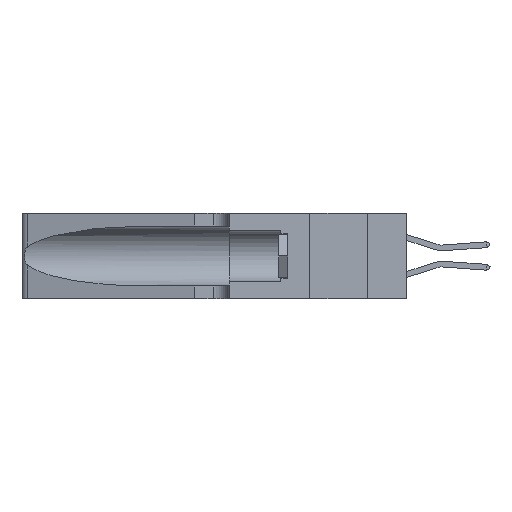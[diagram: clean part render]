
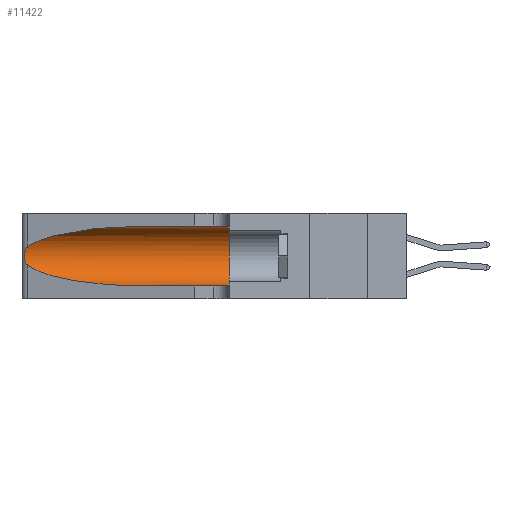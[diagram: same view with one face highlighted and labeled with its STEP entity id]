
A CAD part, left-side view. The second image highlights one B-rep face of the part: STEP entity #11422.
In plain terms, the highlighted cylindrical face has radius 3.308 mm (diameter 6.617 mm), a partial arc.
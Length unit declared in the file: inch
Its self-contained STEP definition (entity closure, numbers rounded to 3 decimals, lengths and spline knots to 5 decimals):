
#431 = CARTESIAN_POINT ( 'NONE',  ( 0.25854, 1.2359, 0.20912 ) ) ;
#1284 = CARTESIAN_POINT ( 'NONE',  ( 0.1305, 0.72297, 0.05475 ) ) ;
#1430 = VERTEX_POINT ( 'NONE', #6978 ) ;
#3313 =( BOUNDED_CURVE ( )  B_SPLINE_CURVE ( 3, ( #6517, #9630, #30344, #12624 ),
 .UNSPECIFIED., .F., .F. ) 
 B_SPLINE_CURVE_WITH_KNOTS ( ( 4, 4 ),
 ( 1.5708, 2.84003 ),
 .UNSPECIFIED. ) 
 CURVE ( )  GEOMETRIC_REPRESENTATION_ITEM ( )  RATIONAL_B_SPLINE_CURVE ( ( 1., 0.87, 0.87, 1. ) ) 
 REPRESENTATION_ITEM ( '' )  );
#3360 = CARTESIAN_POINT ( 'NONE',  ( 0.25487, 1.22718, 0.22369 ) ) ;
#3491 = CARTESIAN_POINT ( 'NONE',  ( 0.26075, 1.23896, 0.19203 ) ) ;
#4408 = B_SPLINE_CURVE_WITH_KNOTS ( 'NONE', 3,
 ( #3360, #15517, #36188, #18493, #431, #21440, #3491, #24396, #6551, #27395, #9664, #30375, #12656, #33358 ),
 .UNSPECIFIED., .F., .F.,
 ( 4, 2, 2, 2, 2, 2, 4 ),
 ( 0., 0.00027, 0.00053, 0.00107, 0.0016, 0.00187, 0.00214 ),
 .UNSPECIFIED. ) ;
#6018 =( BOUNDED_CURVE ( )  B_SPLINE_CURVE ( 3, ( #37023, #16361, #34066, #1284 ),
 .UNSPECIFIED., .F., .T. ) 
 B_SPLINE_CURVE_WITH_KNOTS ( ( 4, 4 ),
 ( 3.44316, 4.71239 ),
 .UNSPECIFIED. ) 
 CURVE ( )  GEOMETRIC_REPRESENTATION_ITEM ( )  RATIONAL_B_SPLINE_CURVE ( ( 1., 0.87, 0.87, 1. ) ) 
 REPRESENTATION_ITEM ( '' )  );
#6517 = CARTESIAN_POINT ( 'NONE',  ( 0.1305, 0.72297, 0.31525 ) ) ;
#6551 = CARTESIAN_POINT ( 'NONE',  ( 0.26017, 1.23833, 0.17102 ) ) ;
#6978 = CARTESIAN_POINT ( 'NONE',  ( 0.1305, 0.35, 0.05475 ) ) ;
#7265 = DIRECTION ( 'NONE',  ( 0., -1., 0. ) ) ;
#9630 = CARTESIAN_POINT ( 'NONE',  ( 0.18966, 0.96281, 0.31525 ) ) ;
#9664 = CARTESIAN_POINT ( 'NONE',  ( 0.25789, 1.23486, 0.15765 ) ) ;
#10448 = ORIENTED_EDGE ( 'NONE', *, *, #18294, .F. ) ;
#11008 = CARTESIAN_POINT ( 'NONE',  ( 0.1305, 0.35, 0.185 ) ) ;
#11091 = CARTESIAN_POINT ( 'NONE',  ( 0.1305, 0.72297, 0.05475 ) ) ;
#11256 = CYLINDRICAL_SURFACE ( 'NONE', #31716, 0.13025 ) ;
#11422 = ADVANCED_FACE ( 'NONE', ( #27886 ), #11256, .F. ) ;
#12431 = VECTOR ( 'NONE', #17589, 39.37008 ) ;
#12624 = CARTESIAN_POINT ( 'NONE',  ( 0.25487, 1.22718, 0.22369 ) ) ;
#12656 = CARTESIAN_POINT ( 'NONE',  ( 0.25555, 1.22993, 0.14849 ) ) ;
#13846 = VERTEX_POINT ( 'NONE', #24570 ) ;
#13916 = VERTEX_POINT ( 'NONE', #16073 ) ;
#13969 = DIRECTION ( 'NONE',  ( 0., 0., 1. ) ) ;
#14313 = LINE ( 'NONE', #35029, #16174 ) ;
#15517 = CARTESIAN_POINT ( 'NONE',  ( 0.25555, 1.22994, 0.2215 ) ) ;
#16073 = CARTESIAN_POINT ( 'NONE',  ( 0.25487, 1.22718, 0.22369 ) ) ;
#16174 = VECTOR ( 'NONE', #20272, 39.37008 ) ;
#16224 = CARTESIAN_POINT ( 'NONE',  ( 0.1305, 1.61858, 0.185 ) ) ;
#16361 = CARTESIAN_POINT ( 'NONE',  ( 0.2373, 1.15595, 0.08982 ) ) ;
#17589 = DIRECTION ( 'NONE',  ( 0., -1., 0. ) ) ;
#18235 = EDGE_CURVE ( 'NONE', #20608, #1430, #14313, .T. ) ;
#18294 = EDGE_CURVE ( 'NONE', #22194, #13846, #20285, .T. ) ;
#18493 = CARTESIAN_POINT ( 'NONE',  ( 0.25787, 1.23484, 0.2124 ) ) ;
#19155 = EDGE_CURVE ( 'NONE', #28384, #20608, #6018, .T. ) ;
#20272 = DIRECTION ( 'NONE',  ( 0., -1., 0. ) ) ;
#20285 = LINE ( 'NONE', #35283, #12431 ) ;
#20608 = VERTEX_POINT ( 'NONE', #11091 ) ;
#21440 = CARTESIAN_POINT ( 'NONE',  ( 0.26018, 1.23835, 0.19895 ) ) ;
#22151 = DIRECTION ( 'NONE',  ( 0., 0., -1. ) ) ;
#22194 = VERTEX_POINT ( 'NONE', #30126 ) ;
#23795 = AXIS2_PLACEMENT_3D ( 'NONE', #11008, #31677, #13969 ) ;
#24085 = EDGE_CURVE ( 'NONE', #13916, #28384, #4408, .T. ) ;
#24396 = CARTESIAN_POINT ( 'NONE',  ( 0.26075, 1.23896, 0.178 ) ) ;
#24570 = CARTESIAN_POINT ( 'NONE',  ( 0.1305, 0.35, 0.31525 ) ) ;
#24674 = EDGE_CURVE ( 'NONE', #22194, #13916, #3313, .T. ) ;
#27395 = CARTESIAN_POINT ( 'NONE',  ( 0.25856, 1.23593, 0.16098 ) ) ;
#27853 = ORIENTED_EDGE ( 'NONE', *, *, #24085, .T. ) ;
#27886 = FACE_OUTER_BOUND ( 'NONE', #31571, .T. ) ;
#28384 = VERTEX_POINT ( 'NONE', #28442 ) ;
#28442 = CARTESIAN_POINT ( 'NONE',  ( 0.25487, 1.22718, 0.14631 ) ) ;
#30126 = CARTESIAN_POINT ( 'NONE',  ( 0.1305, 0.72297, 0.31525 ) ) ;
#30344 = CARTESIAN_POINT ( 'NONE',  ( 0.2373, 1.15595, 0.28018 ) ) ;
#30375 = CARTESIAN_POINT ( 'NONE',  ( 0.25639, 1.23186, 0.15144 ) ) ;
#31571 = EDGE_LOOP ( 'NONE', ( #38139, #27853, #33681, #33706, #35121, #10448 ) ) ;
#31677 = DIRECTION ( 'NONE',  ( 0., 1., 0. ) ) ;
#31716 = AXIS2_PLACEMENT_3D ( 'NONE', #16224, #7265, #22151 ) ;
#33358 = CARTESIAN_POINT ( 'NONE',  ( 0.25487, 1.22718, 0.14631 ) ) ;
#33681 = ORIENTED_EDGE ( 'NONE', *, *, #19155, .T. ) ;
#33706 = ORIENTED_EDGE ( 'NONE', *, *, #18235, .T. ) ;
#34066 = CARTESIAN_POINT ( 'NONE',  ( 0.18966, 0.96281, 0.05475 ) ) ;
#35029 = CARTESIAN_POINT ( 'NONE',  ( 0.1305, 1.61858, 0.05475 ) ) ;
#35121 = ORIENTED_EDGE ( 'NONE', *, *, #37088, .F. ) ;
#35283 = CARTESIAN_POINT ( 'NONE',  ( 0.1305, 1.61858, 0.31525 ) ) ;
#36188 = CARTESIAN_POINT ( 'NONE',  ( 0.25639, 1.23184, 0.21858 ) ) ;
#37023 = CARTESIAN_POINT ( 'NONE',  ( 0.25487, 1.22718, 0.14631 ) ) ;
#37088 = EDGE_CURVE ( 'NONE', #13846, #1430, #38468, .T. ) ;
#38139 = ORIENTED_EDGE ( 'NONE', *, *, #24674, .T. ) ;
#38468 = CIRCLE ( 'NONE', #23795, 0.13025 ) ;
